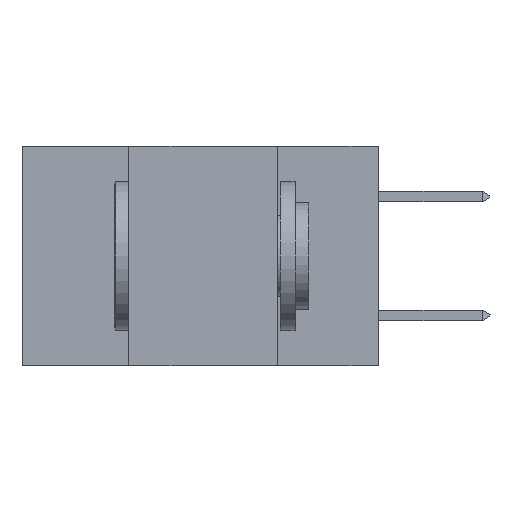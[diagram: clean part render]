
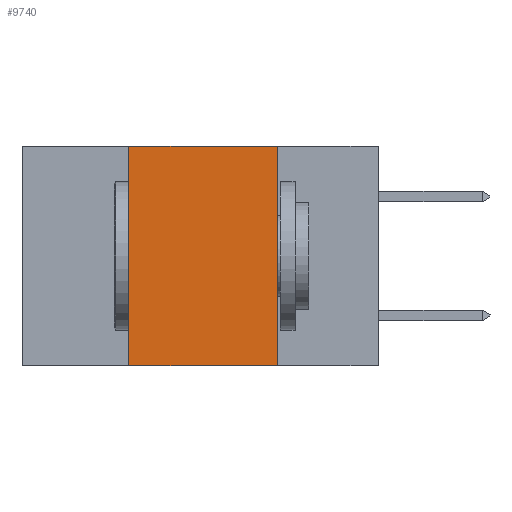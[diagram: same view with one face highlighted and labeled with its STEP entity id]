
A CAD part, left-side view. The second image highlights one B-rep face of the part: STEP entity #9740.
In plain terms, the highlighted planar face has unit normal (-1, 0, 0).
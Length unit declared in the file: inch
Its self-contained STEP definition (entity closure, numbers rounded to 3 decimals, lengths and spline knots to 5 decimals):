
#371 = PLANE ( 'NONE',  #1476 ) ;
#454 = DIRECTION ( 'NONE',  ( 0., 0., -1. ) ) ;
#529 = EDGE_CURVE ( 'NONE', #7777, #1091, #2101, .T. ) ;
#854 = EDGE_CURVE ( 'NONE', #2622, #1091, #9192, .T. ) ;
#1091 = VERTEX_POINT ( 'NONE', #1833 ) ;
#1144 = DIRECTION ( 'NONE',  ( 0., -1., 0. ) ) ;
#1194 = DIRECTION ( 'NONE',  ( 1., 0., 0. ) ) ;
#1476 = AXIS2_PLACEMENT_3D ( 'NONE', #5115, #1194, #3584 ) ;
#1833 = CARTESIAN_POINT ( 'NONE',  ( 0., 0.17, -0.37 ) ) ;
#2101 = LINE ( 'NONE', #5132, #5554 ) ;
#2382 = VERTEX_POINT ( 'NONE', #8822 ) ;
#2622 = VERTEX_POINT ( 'NONE', #8422 ) ;
#2871 = CARTESIAN_POINT ( 'NONE',  ( 0., 0.6, -0.37 ) ) ;
#3329 = ORIENTED_EDGE ( 'NONE', *, *, #5661, .F. ) ;
#3551 = EDGE_LOOP ( 'NONE', ( #9148, #3329, #8288, #8397 ) ) ;
#3584 = DIRECTION ( 'NONE',  ( 0., 0., -1. ) ) ;
#3751 = CARTESIAN_POINT ( 'NONE',  ( 0., 0.17, 0. ) ) ;
#3869 = CARTESIAN_POINT ( 'NONE',  ( 0., 0.42, 0. ) ) ;
#4392 = EDGE_CURVE ( 'NONE', #2622, #2382, #4727, .T. ) ;
#4727 = LINE ( 'NONE', #3869, #6588 ) ;
#4938 = VECTOR ( 'NONE', #8419, 39.37008 ) ;
#5115 = CARTESIAN_POINT ( 'NONE',  ( 0., 0.6, 0. ) ) ;
#5132 = CARTESIAN_POINT ( 'NONE',  ( 0., 0.17, 0. ) ) ;
#5554 = VECTOR ( 'NONE', #454, 39.37008 ) ;
#5634 = CARTESIAN_POINT ( 'NONE',  ( 0., 0.6, 0. ) ) ;
#5661 = EDGE_CURVE ( 'NONE', #2382, #7777, #6444, .T. ) ;
#6444 = LINE ( 'NONE', #5634, #9439 ) ;
#6588 = VECTOR ( 'NONE', #9517, 39.37008 ) ;
#7777 = VERTEX_POINT ( 'NONE', #3751 ) ;
#8288 = ORIENTED_EDGE ( 'NONE', *, *, #4392, .F. ) ;
#8397 = ORIENTED_EDGE ( 'NONE', *, *, #854, .T. ) ;
#8419 = DIRECTION ( 'NONE',  ( 0., -1., 0. ) ) ;
#8422 = CARTESIAN_POINT ( 'NONE',  ( 0., 0.42, -0.37 ) ) ;
#8822 = CARTESIAN_POINT ( 'NONE',  ( 0., 0.42, 0. ) ) ;
#9148 = ORIENTED_EDGE ( 'NONE', *, *, #529, .F. ) ;
#9161 = FACE_OUTER_BOUND ( 'NONE', #3551, .T. ) ;
#9192 = LINE ( 'NONE', #2871, #4938 ) ;
#9439 = VECTOR ( 'NONE', #1144, 39.37008 ) ;
#9517 = DIRECTION ( 'NONE',  ( 0., 0., 1. ) ) ;
#9740 = ADVANCED_FACE ( 'NONE', ( #9161 ), #371, .F. ) ;
